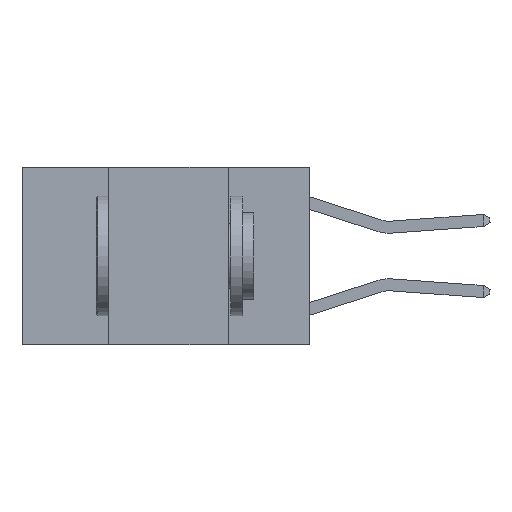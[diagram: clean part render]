
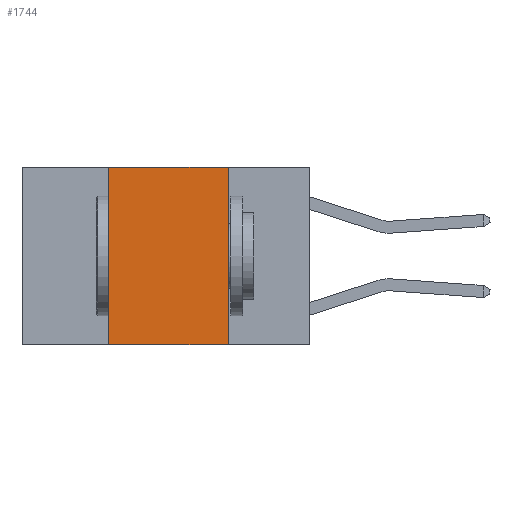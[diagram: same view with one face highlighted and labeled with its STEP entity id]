
A CAD part, left-side view. The second image highlights one B-rep face of the part: STEP entity #1744.
In plain terms, the highlighted planar face has unit normal (-1, 0, 0).
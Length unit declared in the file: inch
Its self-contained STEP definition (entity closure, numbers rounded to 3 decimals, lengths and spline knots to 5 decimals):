
#381 = LINE ( 'NONE', #8555, #4393 ) ;
#455 = CARTESIAN_POINT ( 'NONE',  ( 0., 0.17, 0. ) ) ;
#1011 = CARTESIAN_POINT ( 'NONE',  ( 0., 0.6, 0. ) ) ;
#1743 = DIRECTION ( 'NONE',  ( 0., 0., 1. ) ) ;
#1744 = ADVANCED_FACE ( 'NONE', ( #5351 ), #8328, .F. ) ;
#1796 = LINE ( 'NONE', #8121, #4983 ) ;
#1872 = AXIS2_PLACEMENT_3D ( 'NONE', #1011, #3183, #4047 ) ;
#2194 = VERTEX_POINT ( 'NONE', #2978 ) ;
#2583 = CARTESIAN_POINT ( 'NONE',  ( 0., 0.42, -0.37 ) ) ;
#2665 = EDGE_CURVE ( 'NONE', #7046, #5800, #8875, .T. ) ;
#2782 = ORIENTED_EDGE ( 'NONE', *, *, #3498, .F. ) ;
#2960 = EDGE_CURVE ( 'NONE', #7046, #2194, #11103, .T. ) ;
#2978 = CARTESIAN_POINT ( 'NONE',  ( 0., 0.17, -0.37 ) ) ;
#3183 = DIRECTION ( 'NONE',  ( 1., 0., 0. ) ) ;
#3409 = VERTEX_POINT ( 'NONE', #455 ) ;
#3498 = EDGE_CURVE ( 'NONE', #5800, #3409, #381, .T. ) ;
#4047 = DIRECTION ( 'NONE',  ( 0., 0., -1. ) ) ;
#4393 = VECTOR ( 'NONE', #11664, 39.37008 ) ;
#4486 = ORIENTED_EDGE ( 'NONE', *, *, #8079, .F. ) ;
#4983 = VECTOR ( 'NONE', #7002, 39.37008 ) ;
#5351 = FACE_OUTER_BOUND ( 'NONE', #11959, .T. ) ;
#5800 = VERTEX_POINT ( 'NONE', #9426 ) ;
#5876 = DIRECTION ( 'NONE',  ( 0., -1., 0. ) ) ;
#6438 = VECTOR ( 'NONE', #5876, 39.37008 ) ;
#6925 = ORIENTED_EDGE ( 'NONE', *, *, #2665, .F. ) ;
#7002 = DIRECTION ( 'NONE',  ( 0., 0., -1. ) ) ;
#7046 = VERTEX_POINT ( 'NONE', #2583 ) ;
#7959 = CARTESIAN_POINT ( 'NONE',  ( 0., 0.6, -0.37 ) ) ;
#8079 = EDGE_CURVE ( 'NONE', #3409, #2194, #1796, .T. ) ;
#8121 = CARTESIAN_POINT ( 'NONE',  ( 0., 0.17, 0. ) ) ;
#8328 = PLANE ( 'NONE',  #1872 ) ;
#8555 = CARTESIAN_POINT ( 'NONE',  ( 0., 0.6, 0. ) ) ;
#8875 = LINE ( 'NONE', #9980, #13034 ) ;
#9426 = CARTESIAN_POINT ( 'NONE',  ( 0., 0.42, 0. ) ) ;
#9947 = ORIENTED_EDGE ( 'NONE', *, *, #2960, .T. ) ;
#9980 = CARTESIAN_POINT ( 'NONE',  ( 0., 0.42, 0. ) ) ;
#11103 = LINE ( 'NONE', #7959, #6438 ) ;
#11664 = DIRECTION ( 'NONE',  ( 0., -1., 0. ) ) ;
#11959 = EDGE_LOOP ( 'NONE', ( #4486, #2782, #6925, #9947 ) ) ;
#13034 = VECTOR ( 'NONE', #1743, 39.37008 ) ;
